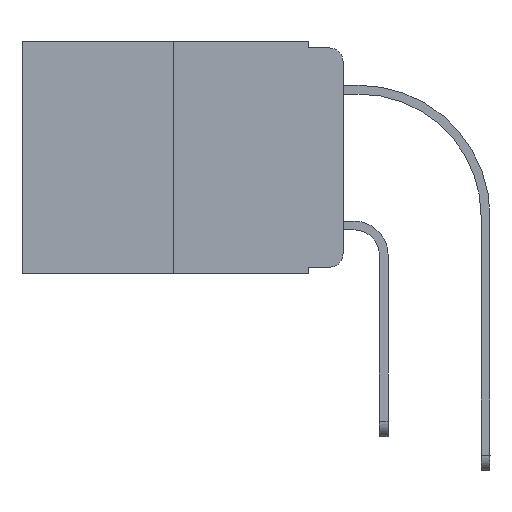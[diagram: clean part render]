
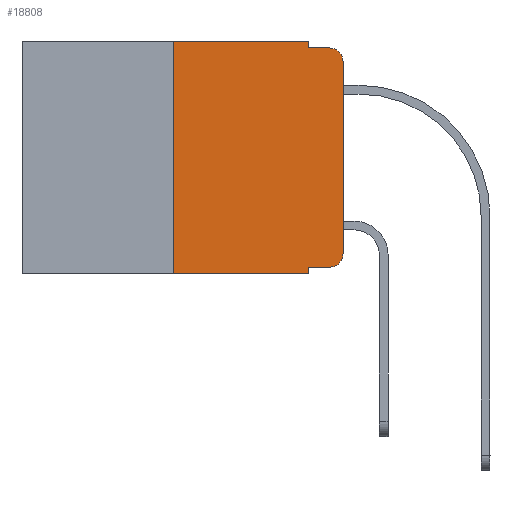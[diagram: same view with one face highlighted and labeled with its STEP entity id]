
A CAD part, left-side view. The second image highlights one B-rep face of the part: STEP entity #18808.
In plain terms, the highlighted planar face has unit normal (-1, 0, 0).
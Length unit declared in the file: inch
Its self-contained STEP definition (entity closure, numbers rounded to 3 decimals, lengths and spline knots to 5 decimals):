
#411 = VECTOR ( 'NONE', #19419, 39.37008 ) ;
#664 = CARTESIAN_POINT ( 'NONE',  ( 0., 0.051, -0.01 ) ) ;
#709 = PLANE ( 'NONE',  #10219 ) ;
#839 = CARTESIAN_POINT ( 'NONE',  ( 0., 0.25, -0.343 ) ) ;
#850 = ORIENTED_EDGE ( 'NONE', *, *, #22722, .F. ) ;
#1444 = VERTEX_POINT ( 'NONE', #15451 ) ;
#1679 = EDGE_CURVE ( 'NONE', #9399, #23892, #6555, .T. ) ;
#1703 = VECTOR ( 'NONE', #4279, 39.37008 ) ;
#1835 = CARTESIAN_POINT ( 'NONE',  ( 0., 0.051, -0.01 ) ) ;
#3152 = LINE ( 'NONE', #15147, #18577 ) ;
#3352 = ORIENTED_EDGE ( 'NONE', *, *, #1679, .F. ) ;
#3441 = EDGE_CURVE ( 'NONE', #11912, #23942, #8620, .T. ) ;
#3966 = VERTEX_POINT ( 'NONE', #21099 ) ;
#4279 = DIRECTION ( 'NONE',  ( 0., -1., 0. ) ) ;
#4800 = CARTESIAN_POINT ( 'NONE',  ( 0., 0.02, -0.313 ) ) ;
#5221 = CARTESIAN_POINT ( 'NONE',  ( 0., 0.02, -0.03 ) ) ;
#5911 = ORIENTED_EDGE ( 'NONE', *, *, #23284, .T. ) ;
#6011 = CARTESIAN_POINT ( 'NONE',  ( 0., 0.051, 0. ) ) ;
#6404 = CARTESIAN_POINT ( 'NONE',  ( 0., 0.02, -0.333 ) ) ;
#6555 = LINE ( 'NONE', #664, #22166 ) ;
#6636 = AXIS2_PLACEMENT_3D ( 'NONE', #5221, #14998, #16832 ) ;
#6919 = ORIENTED_EDGE ( 'NONE', *, *, #23567, .T. ) ;
#8167 = LINE ( 'NONE', #12064, #24599 ) ;
#8273 = EDGE_LOOP ( 'NONE', ( #20506, #13202, #3352, #850, #21717, #20099, #6919, #15416, #5911, #21751 ) ) ;
#8620 = LINE ( 'NONE', #16449, #12495 ) ;
#8881 = DIRECTION ( 'NONE',  ( 0., 0., 1. ) ) ;
#9399 = VERTEX_POINT ( 'NONE', #1835 ) ;
#9682 = LINE ( 'NONE', #17880, #17132 ) ;
#10219 = AXIS2_PLACEMENT_3D ( 'NONE', #24601, #14690, #15721 ) ;
#10269 = EDGE_CURVE ( 'NONE', #19523, #1444, #21467, .T. ) ;
#10612 = DIRECTION ( 'NONE',  ( 0., -1., 0. ) ) ;
#11912 = VERTEX_POINT ( 'NONE', #839 ) ;
#11965 = VERTEX_POINT ( 'NONE', #15216 ) ;
#12064 = CARTESIAN_POINT ( 'NONE',  ( 0., 0.473, -0.343 ) ) ;
#12495 = VECTOR ( 'NONE', #8881, 39.37008 ) ;
#12763 = DIRECTION ( 'NONE',  ( 0., 0., -1. ) ) ;
#12993 = CARTESIAN_POINT ( 'NONE',  ( 0., 0., -0.03 ) ) ;
#13202 = ORIENTED_EDGE ( 'NONE', *, *, #22935, .T. ) ;
#13776 = EDGE_CURVE ( 'NONE', #1444, #20064, #3152, .T. ) ;
#13966 = DIRECTION ( 'NONE',  ( 0., 0., -1. ) ) ;
#14690 = DIRECTION ( 'NONE',  ( 1., 0., 0. ) ) ;
#14998 = DIRECTION ( 'NONE',  ( -1., 0., 0. ) ) ;
#15147 = CARTESIAN_POINT ( 'NONE',  ( 0., 0., 0. ) ) ;
#15216 = CARTESIAN_POINT ( 'NONE',  ( 0., 0.051, -0.343 ) ) ;
#15416 = ORIENTED_EDGE ( 'NONE', *, *, #21307, .F. ) ;
#15451 = CARTESIAN_POINT ( 'NONE',  ( 0., 0., -0.313 ) ) ;
#15721 = DIRECTION ( 'NONE',  ( 0., 0., -1. ) ) ;
#16449 = CARTESIAN_POINT ( 'NONE',  ( 0., 0.25, 0. ) ) ;
#16729 = DIRECTION ( 'NONE',  ( 0., -1., 0. ) ) ;
#16735 = CARTESIAN_POINT ( 'NONE',  ( 0., 0.051, -0.333 ) ) ;
#16832 = DIRECTION ( 'NONE',  ( 0., 0., -1. ) ) ;
#17132 = VECTOR ( 'NONE', #21789, 39.37008 ) ;
#17164 = EDGE_CURVE ( 'NONE', #23942, #3966, #23455, .T. ) ;
#17880 = CARTESIAN_POINT ( 'NONE',  ( 0., 0.051, 0. ) ) ;
#18371 = LINE ( 'NONE', #22147, #1703 ) ;
#18577 = VECTOR ( 'NONE', #22836, 39.37008 ) ;
#18760 = DIRECTION ( 'NONE',  ( -1., 0., 0. ) ) ;
#18808 = ADVANCED_FACE ( 'NONE', ( #20560 ), #709, .F. ) ;
#18988 = AXIS2_PLACEMENT_3D ( 'NONE', #4800, #18760, #12763 ) ;
#19419 = DIRECTION ( 'NONE',  ( 0., -1., 0. ) ) ;
#19523 = VERTEX_POINT ( 'NONE', #6404 ) ;
#20064 = VERTEX_POINT ( 'NONE', #12993 ) ;
#20099 = ORIENTED_EDGE ( 'NONE', *, *, #3441, .F. ) ;
#20109 = CARTESIAN_POINT ( 'NONE',  ( 0., 0.25, 0. ) ) ;
#20506 = ORIENTED_EDGE ( 'NONE', *, *, #13776, .T. ) ;
#20560 = FACE_OUTER_BOUND ( 'NONE', #8273, .T. ) ;
#21099 = CARTESIAN_POINT ( 'NONE',  ( 0., 0.051, 0. ) ) ;
#21227 = VECTOR ( 'NONE', #13966, 39.37008 ) ;
#21307 = EDGE_CURVE ( 'NONE', #22396, #11965, #9682, .T. ) ;
#21467 = CIRCLE ( 'NONE', #18988, 0.02 ) ;
#21717 = ORIENTED_EDGE ( 'NONE', *, *, #17164, .F. ) ;
#21751 = ORIENTED_EDGE ( 'NONE', *, *, #10269, .T. ) ;
#21789 = DIRECTION ( 'NONE',  ( 0., 0., -1. ) ) ;
#22043 = CARTESIAN_POINT ( 'NONE',  ( 0., 0.02, -0.01 ) ) ;
#22147 = CARTESIAN_POINT ( 'NONE',  ( 0., 0.051, -0.333 ) ) ;
#22166 = VECTOR ( 'NONE', #16729, 39.37008 ) ;
#22396 = VERTEX_POINT ( 'NONE', #16735 ) ;
#22722 = EDGE_CURVE ( 'NONE', #3966, #9399, #23889, .T. ) ;
#22836 = DIRECTION ( 'NONE',  ( 0., 0., 1. ) ) ;
#22904 = CIRCLE ( 'NONE', #6636, 0.02 ) ;
#22935 = EDGE_CURVE ( 'NONE', #20064, #23892, #22904, .T. ) ;
#23284 = EDGE_CURVE ( 'NONE', #22396, #19523, #18371, .T. ) ;
#23455 = LINE ( 'NONE', #23696, #411 ) ;
#23567 = EDGE_CURVE ( 'NONE', #11912, #11965, #8167, .T. ) ;
#23696 = CARTESIAN_POINT ( 'NONE',  ( 0., 0.473, 0. ) ) ;
#23889 = LINE ( 'NONE', #6011, #21227 ) ;
#23892 = VERTEX_POINT ( 'NONE', #22043 ) ;
#23942 = VERTEX_POINT ( 'NONE', #20109 ) ;
#24599 = VECTOR ( 'NONE', #10612, 39.37008 ) ;
#24601 = CARTESIAN_POINT ( 'NONE',  ( 0., 0.473, 0. ) ) ;
